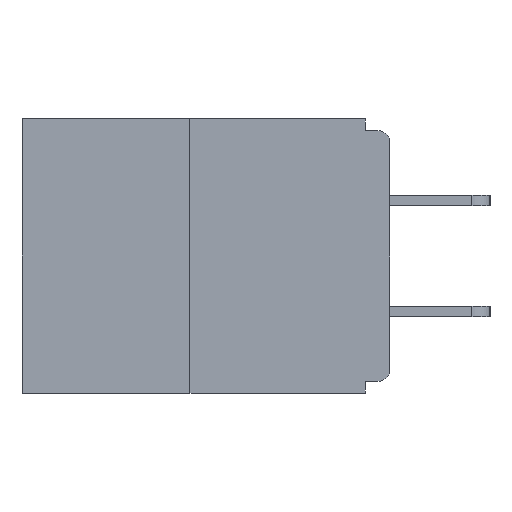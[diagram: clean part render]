
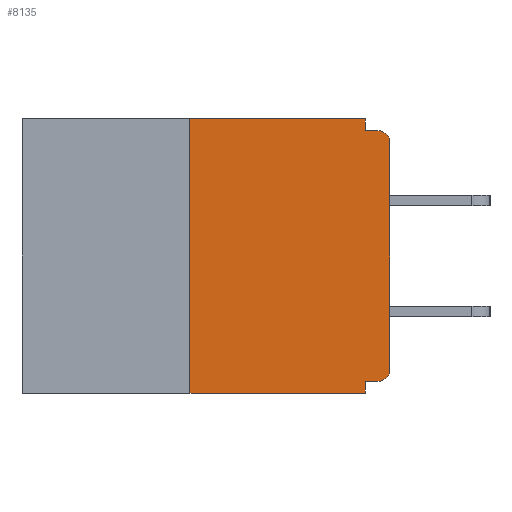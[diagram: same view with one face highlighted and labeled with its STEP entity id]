
A CAD part, left-side view. The second image highlights one B-rep face of the part: STEP entity #8135.
In plain terms, the highlighted planar face has unit normal (-1, 0, 0).
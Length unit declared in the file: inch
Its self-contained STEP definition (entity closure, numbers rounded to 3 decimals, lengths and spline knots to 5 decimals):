
#344 = ORIENTED_EDGE ( 'NONE', *, *, #4809, .T. ) ;
#369 = LINE ( 'NONE', #430, #4942 ) ;
#430 = CARTESIAN_POINT ( 'NONE',  ( 0., 0.031, -0.343 ) ) ;
#605 = VECTOR ( 'NONE', #3064, 39.37008 ) ;
#697 = DIRECTION ( 'NONE',  ( 0., 0., -1. ) ) ;
#704 = EDGE_CURVE ( 'NONE', #6471, #5276, #11120, .T. ) ;
#762 = CARTESIAN_POINT ( 'NONE',  ( 0., 0.015, -0.015 ) ) ;
#813 = DIRECTION ( 'NONE',  ( 0., 0., 1. ) ) ;
#858 = DIRECTION ( 'NONE',  ( 0., -1., 0. ) ) ;
#906 = DIRECTION ( 'NONE',  ( 0., 0., 1. ) ) ;
#907 = DIRECTION ( 'NONE',  ( 0., 0., -1. ) ) ;
#984 = EDGE_CURVE ( 'NONE', #6471, #7143, #1867, .T. ) ;
#1121 = ORIENTED_EDGE ( 'NONE', *, *, #7922, .F. ) ;
#1381 = CARTESIAN_POINT ( 'NONE',  ( 0., 0.031, -0.328 ) ) ;
#1657 = ORIENTED_EDGE ( 'NONE', *, *, #8570, .T. ) ;
#1867 = LINE ( 'NONE', #3407, #12375 ) ;
#1894 = CARTESIAN_POINT ( 'NONE',  ( 0., 0.46, -0.343 ) ) ;
#2338 = LINE ( 'NONE', #9199, #10956 ) ;
#2668 = EDGE_CURVE ( 'NONE', #11808, #5769, #2338, .T. ) ;
#2696 = ORIENTED_EDGE ( 'NONE', *, *, #5846, .T. ) ;
#3064 = DIRECTION ( 'NONE',  ( 0., -1., 0. ) ) ;
#3180 = CARTESIAN_POINT ( 'NONE',  ( 0., 0.031, -0.015 ) ) ;
#3407 = CARTESIAN_POINT ( 'NONE',  ( 0., 0.25, 0. ) ) ;
#3467 = VECTOR ( 'NONE', #858, 39.37008 ) ;
#3884 = CARTESIAN_POINT ( 'NONE',  ( 0., 0., -0.313 ) ) ;
#4319 = CARTESIAN_POINT ( 'NONE',  ( 0., 0., -0.328 ) ) ;
#4713 = AXIS2_PLACEMENT_3D ( 'NONE', #12596, #8424, #12661 ) ;
#4740 = VERTEX_POINT ( 'NONE', #3884 ) ;
#4809 = EDGE_CURVE ( 'NONE', #4740, #10323, #5813, .T. ) ;
#4942 = VECTOR ( 'NONE', #7646, 39.37008 ) ;
#5017 = DIRECTION ( 'NONE',  ( 0., -1., 0. ) ) ;
#5259 = EDGE_CURVE ( 'NONE', #7143, #11808, #8242, .T. ) ;
#5276 = VERTEX_POINT ( 'NONE', #9178 ) ;
#5344 = CIRCLE ( 'NONE', #4713, 0.015 ) ;
#5769 = VERTEX_POINT ( 'NONE', #3180 ) ;
#5813 = LINE ( 'NONE', #12105, #11843 ) ;
#5846 = EDGE_CURVE ( 'NONE', #11812, #4740, #5344, .T. ) ;
#5942 = CARTESIAN_POINT ( 'NONE',  ( 0., 0.015, -0.03 ) ) ;
#6283 = CARTESIAN_POINT ( 'NONE',  ( 0., 0.46, 0. ) ) ;
#6408 = CARTESIAN_POINT ( 'NONE',  ( 0., 0.015, -0.328 ) ) ;
#6471 = VERTEX_POINT ( 'NONE', #6988 ) ;
#6633 = CIRCLE ( 'NONE', #10879, 0.015 ) ;
#6932 = EDGE_CURVE ( 'NONE', #10079, #5276, #369, .T. ) ;
#6988 = CARTESIAN_POINT ( 'NONE',  ( 0., 0.25, -0.343 ) ) ;
#7076 = VERTEX_POINT ( 'NONE', #762 ) ;
#7116 = EDGE_CURVE ( 'NONE', #11812, #10079, #11419, .T. ) ;
#7143 = VERTEX_POINT ( 'NONE', #12287 ) ;
#7258 = ORIENTED_EDGE ( 'NONE', *, *, #5259, .F. ) ;
#7646 = DIRECTION ( 'NONE',  ( 0., 0., -1. ) ) ;
#7648 = DIRECTION ( 'NONE',  ( 1., 0., 0. ) ) ;
#7922 = EDGE_CURVE ( 'NONE', #5769, #7076, #12799, .T. ) ;
#8135 = ADVANCED_FACE ( 'NONE', ( #9585 ), #11701, .F. ) ;
#8242 = LINE ( 'NONE', #10231, #605 ) ;
#8309 = DIRECTION ( 'NONE',  ( 0., 1., 0. ) ) ;
#8424 = DIRECTION ( 'NONE',  ( -1., 0., 0. ) ) ;
#8544 = EDGE_LOOP ( 'NONE', ( #7258, #12202, #10779, #10523, #12755, #2696, #344, #1657, #1121, #9402 ) ) ;
#8570 = EDGE_CURVE ( 'NONE', #10323, #7076, #6633, .T. ) ;
#9126 = VECTOR ( 'NONE', #5017, 39.37008 ) ;
#9178 = CARTESIAN_POINT ( 'NONE',  ( 0., 0.031, -0.343 ) ) ;
#9199 = CARTESIAN_POINT ( 'NONE',  ( 0., 0.031, 0. ) ) ;
#9402 = ORIENTED_EDGE ( 'NONE', *, *, #2668, .F. ) ;
#9585 = FACE_OUTER_BOUND ( 'NONE', #8544, .T. ) ;
#9994 = DIRECTION ( 'NONE',  ( -1., 0., 0. ) ) ;
#10079 = VERTEX_POINT ( 'NONE', #1381 ) ;
#10194 = CARTESIAN_POINT ( 'NONE',  ( 0., 0., -0.03 ) ) ;
#10231 = CARTESIAN_POINT ( 'NONE',  ( 0., 0.46, 0. ) ) ;
#10323 = VERTEX_POINT ( 'NONE', #10194 ) ;
#10523 = ORIENTED_EDGE ( 'NONE', *, *, #6932, .F. ) ;
#10779 = ORIENTED_EDGE ( 'NONE', *, *, #704, .T. ) ;
#10879 = AXIS2_PLACEMENT_3D ( 'NONE', #5942, #9994, #907 ) ;
#10956 = VECTOR ( 'NONE', #11180, 39.37008 ) ;
#11120 = LINE ( 'NONE', #1894, #9126 ) ;
#11180 = DIRECTION ( 'NONE',  ( 0., 0., -1. ) ) ;
#11419 = LINE ( 'NONE', #4319, #13044 ) ;
#11701 = PLANE ( 'NONE',  #12807 ) ;
#11803 = CARTESIAN_POINT ( 'NONE',  ( 0., 0., -0.015 ) ) ;
#11808 = VERTEX_POINT ( 'NONE', #12318 ) ;
#11812 = VERTEX_POINT ( 'NONE', #6408 ) ;
#11843 = VECTOR ( 'NONE', #906, 39.37008 ) ;
#12105 = CARTESIAN_POINT ( 'NONE',  ( 0., 0., 0. ) ) ;
#12202 = ORIENTED_EDGE ( 'NONE', *, *, #984, .F. ) ;
#12287 = CARTESIAN_POINT ( 'NONE',  ( 0., 0.25, 0. ) ) ;
#12318 = CARTESIAN_POINT ( 'NONE',  ( 0., 0.031, 0. ) ) ;
#12375 = VECTOR ( 'NONE', #813, 39.37008 ) ;
#12596 = CARTESIAN_POINT ( 'NONE',  ( 0., 0.015, -0.313 ) ) ;
#12661 = DIRECTION ( 'NONE',  ( 0., 0., -1. ) ) ;
#12755 = ORIENTED_EDGE ( 'NONE', *, *, #7116, .F. ) ;
#12799 = LINE ( 'NONE', #11803, #3467 ) ;
#12807 = AXIS2_PLACEMENT_3D ( 'NONE', #6283, #7648, #697 ) ;
#13044 = VECTOR ( 'NONE', #8309, 39.37008 ) ;
